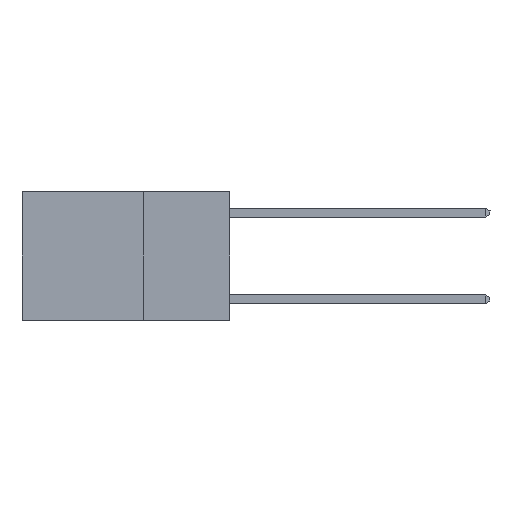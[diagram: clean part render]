
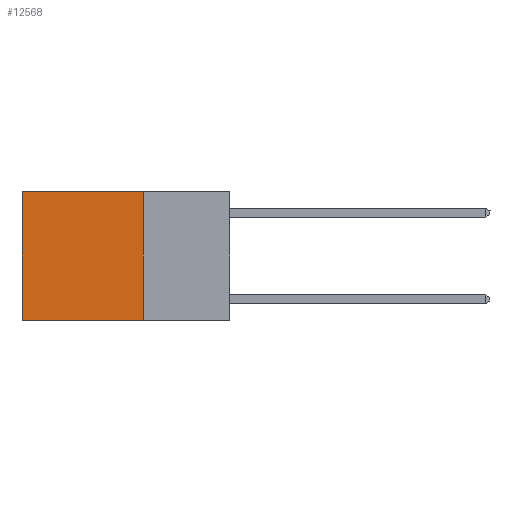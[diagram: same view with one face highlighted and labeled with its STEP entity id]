
A CAD part, left-side view. The second image highlights one B-rep face of the part: STEP entity #12568.
In plain terms, the highlighted planar face has unit normal (-1, 0, 0).
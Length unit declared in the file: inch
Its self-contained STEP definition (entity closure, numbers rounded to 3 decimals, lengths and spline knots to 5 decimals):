
#80 = EDGE_CURVE ( 'NONE', #3539, #2029, #6460, .T. ) ;
#249 = AXIS2_PLACEMENT_3D ( 'NONE', #7860, #8132, #13134 ) ;
#343 = VERTEX_POINT ( 'NONE', #2448 ) ;
#928 = DIRECTION ( 'NONE',  ( 0., 0., -1. ) ) ;
#1116 = ORIENTED_EDGE ( 'NONE', *, *, #2960, .F. ) ;
#1318 = VECTOR ( 'NONE', #928, 39.37008 ) ;
#1612 = VECTOR ( 'NONE', #3973, 39.37008 ) ;
#2029 = VERTEX_POINT ( 'NONE', #5654 ) ;
#2329 = VERTEX_POINT ( 'NONE', #2939 ) ;
#2440 = CARTESIAN_POINT ( 'NONE',  ( 0.2625, 0.6, 0. ) ) ;
#2448 = CARTESIAN_POINT ( 'NONE',  ( 0.2625, 0.25, 0. ) ) ;
#2939 = CARTESIAN_POINT ( 'NONE',  ( 0.2625, 0.6, 0. ) ) ;
#2960 = EDGE_CURVE ( 'NONE', #343, #3539, #9125, .T. ) ;
#3529 = LINE ( 'NONE', #2440, #7466 ) ;
#3539 = VERTEX_POINT ( 'NONE', #11621 ) ;
#3973 = DIRECTION ( 'NONE',  ( 0., 1., 0. ) ) ;
#4097 = LINE ( 'NONE', #8179, #1612 ) ;
#4729 = EDGE_CURVE ( 'NONE', #343, #2329, #4097, .T. ) ;
#5654 = CARTESIAN_POINT ( 'NONE',  ( 0.2625, 0.6, -0.37 ) ) ;
#6460 = LINE ( 'NONE', #8746, #11810 ) ;
#7466 = VECTOR ( 'NONE', #10734, 39.37008 ) ;
#7860 = CARTESIAN_POINT ( 'NONE',  ( 0.2625, 0.25, 0. ) ) ;
#8109 = EDGE_LOOP ( 'NONE', ( #12369, #10937, #1116, #12156 ) ) ;
#8132 = DIRECTION ( 'NONE',  ( 1., 0., 0. ) ) ;
#8179 = CARTESIAN_POINT ( 'NONE',  ( 0.2625, 0.25, 0. ) ) ;
#8263 = EDGE_CURVE ( 'NONE', #2329, #2029, #3529, .T. ) ;
#8746 = CARTESIAN_POINT ( 'NONE',  ( 0.2625, 0.25, -0.37 ) ) ;
#8996 = FACE_OUTER_BOUND ( 'NONE', #8109, .T. ) ;
#9125 = LINE ( 'NONE', #12307, #1318 ) ;
#10595 = DIRECTION ( 'NONE',  ( 0., 1., 0. ) ) ;
#10734 = DIRECTION ( 'NONE',  ( 0., 0., -1. ) ) ;
#10937 = ORIENTED_EDGE ( 'NONE', *, *, #80, .F. ) ;
#11621 = CARTESIAN_POINT ( 'NONE',  ( 0.2625, 0.25, -0.37 ) ) ;
#11810 = VECTOR ( 'NONE', #10595, 39.37008 ) ;
#12156 = ORIENTED_EDGE ( 'NONE', *, *, #4729, .T. ) ;
#12307 = CARTESIAN_POINT ( 'NONE',  ( 0.2625, 0.25, 0. ) ) ;
#12369 = ORIENTED_EDGE ( 'NONE', *, *, #8263, .T. ) ;
#12568 = ADVANCED_FACE ( 'NONE', ( #8996 ), #13248, .F. ) ;
#13134 = DIRECTION ( 'NONE',  ( 0., 0., -1. ) ) ;
#13248 = PLANE ( 'NONE',  #249 ) ;
